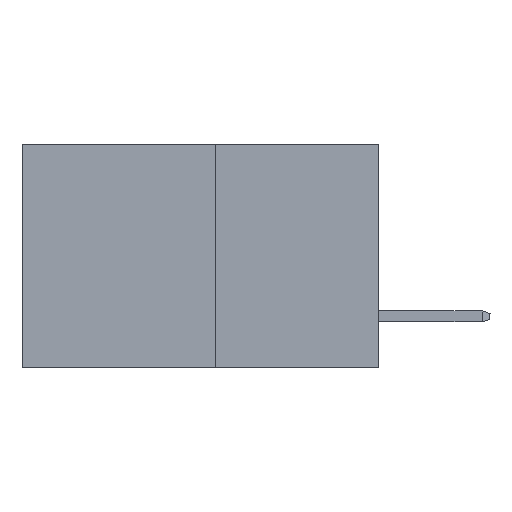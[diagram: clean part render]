
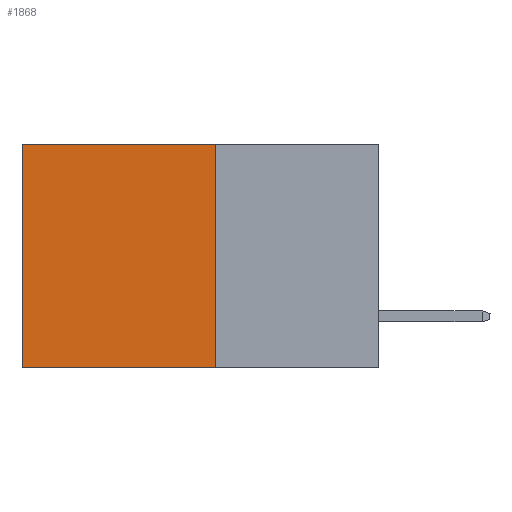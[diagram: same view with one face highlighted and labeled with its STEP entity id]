
A CAD part, left-side view. The second image highlights one B-rep face of the part: STEP entity #1868.
In plain terms, the highlighted planar face has unit normal (-1, 0, 0).
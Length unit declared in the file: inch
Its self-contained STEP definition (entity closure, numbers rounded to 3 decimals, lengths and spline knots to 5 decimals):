
#832 = VECTOR ( 'NONE', #11006, 39.37008 ) ;
#1742 = FACE_OUTER_BOUND ( 'NONE', #4189, .T. ) ;
#1868 = ADVANCED_FACE ( 'NONE', ( #1742 ), #11691, .F. ) ;
#2210 = CARTESIAN_POINT ( 'NONE',  ( 0.277, 0.27, -0.37 ) ) ;
#2493 = EDGE_CURVE ( 'NONE', #10624, #10562, #5540, .T. ) ;
#3831 = VERTEX_POINT ( 'NONE', #6964 ) ;
#4189 = EDGE_LOOP ( 'NONE', ( #8073, #7901, #8390, #4821 ) ) ;
#4275 = VECTOR ( 'NONE', #9328, 39.37008 ) ;
#4547 = CARTESIAN_POINT ( 'NONE',  ( 0.277, 0.59, -0.37 ) ) ;
#4821 = ORIENTED_EDGE ( 'NONE', *, *, #6895, .T. ) ;
#5540 = LINE ( 'NONE', #10317, #6211 ) ;
#6211 = VECTOR ( 'NONE', #10840, 39.37008 ) ;
#6693 = LINE ( 'NONE', #2210, #832 ) ;
#6895 = EDGE_CURVE ( 'NONE', #10624, #3831, #7208, .T. ) ;
#6964 = CARTESIAN_POINT ( 'NONE',  ( 0.277, 0.59, 0. ) ) ;
#7208 = LINE ( 'NONE', #11450, #4275 ) ;
#7651 = LINE ( 'NONE', #4547, #10535 ) ;
#7901 = ORIENTED_EDGE ( 'NONE', *, *, #11308, .F. ) ;
#8073 = ORIENTED_EDGE ( 'NONE', *, *, #8901, .T. ) ;
#8390 = ORIENTED_EDGE ( 'NONE', *, *, #2493, .F. ) ;
#8901 = EDGE_CURVE ( 'NONE', #3831, #8985, #7651, .T. ) ;
#8914 = DIRECTION ( 'NONE',  ( 0., 0., -1. ) ) ;
#8985 = VERTEX_POINT ( 'NONE', #13430 ) ;
#9328 = DIRECTION ( 'NONE',  ( 0., 1., 0. ) ) ;
#9439 = AXIS2_PLACEMENT_3D ( 'NONE', #13203, #11487, #11470 ) ;
#10317 = CARTESIAN_POINT ( 'NONE',  ( 0.277, 0.27, -0.37 ) ) ;
#10535 = VECTOR ( 'NONE', #8914, 39.37008 ) ;
#10562 = VERTEX_POINT ( 'NONE', #13195 ) ;
#10624 = VERTEX_POINT ( 'NONE', #13342 ) ;
#10840 = DIRECTION ( 'NONE',  ( 0., 0., -1. ) ) ;
#11006 = DIRECTION ( 'NONE',  ( 0., 1., 0. ) ) ;
#11308 = EDGE_CURVE ( 'NONE', #10562, #8985, #6693, .T. ) ;
#11450 = CARTESIAN_POINT ( 'NONE',  ( 0.277, 0.27, 0. ) ) ;
#11470 = DIRECTION ( 'NONE',  ( 0., 0., -1. ) ) ;
#11487 = DIRECTION ( 'NONE',  ( 1., 0., 0. ) ) ;
#11691 = PLANE ( 'NONE',  #9439 ) ;
#13195 = CARTESIAN_POINT ( 'NONE',  ( 0.277, 0.27, -0.37 ) ) ;
#13203 = CARTESIAN_POINT ( 'NONE',  ( 0.277, 0.27, -0.37 ) ) ;
#13342 = CARTESIAN_POINT ( 'NONE',  ( 0.277, 0.27, 0. ) ) ;
#13430 = CARTESIAN_POINT ( 'NONE',  ( 0.277, 0.59, -0.37 ) ) ;
